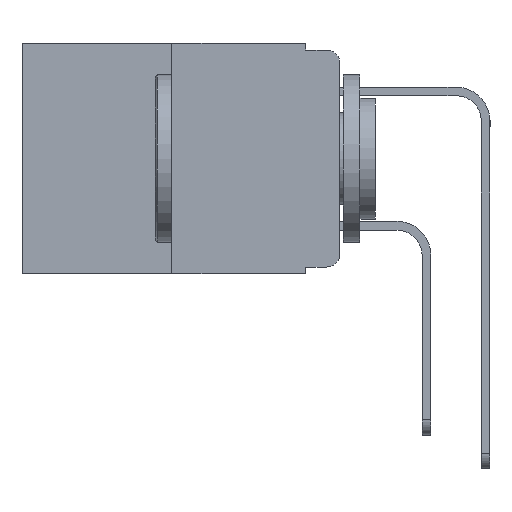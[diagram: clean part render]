
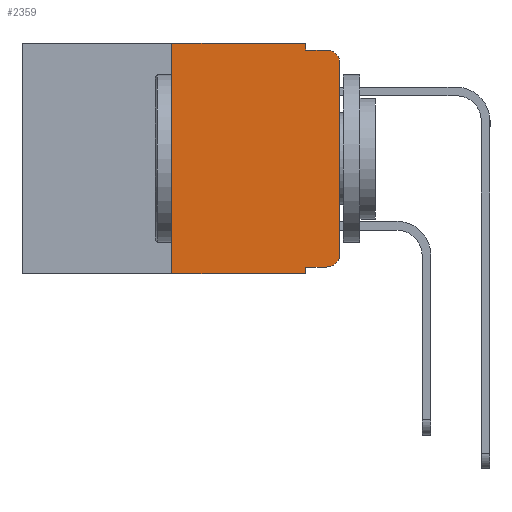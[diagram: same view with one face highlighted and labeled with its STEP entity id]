
A CAD part, left-side view. The second image highlights one B-rep face of the part: STEP entity #2359.
In plain terms, the highlighted planar face has unit normal (-1, 0, 0).
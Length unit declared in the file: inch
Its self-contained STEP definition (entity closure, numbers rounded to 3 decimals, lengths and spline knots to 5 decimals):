
#5 = CARTESIAN_POINT ( 'NONE',  ( 0., 0.051, -0.333 ) ) ;
#31 = VERTEX_POINT ( 'NONE', #13778 ) ;
#404 = LINE ( 'NONE', #16839, #7395 ) ;
#1077 = CARTESIAN_POINT ( 'NONE',  ( 0., 0.02, -0.333 ) ) ;
#1206 = ORIENTED_EDGE ( 'NONE', *, *, #13495, .T. ) ;
#1673 = VERTEX_POINT ( 'NONE', #5 ) ;
#1709 = VERTEX_POINT ( 'NONE', #17015 ) ;
#1797 = CARTESIAN_POINT ( 'NONE',  ( 0., 0.25, -0.343 ) ) ;
#1930 = VERTEX_POINT ( 'NONE', #12242 ) ;
#2124 = EDGE_CURVE ( 'NONE', #31, #9422, #9841, .T. ) ;
#2218 = CIRCLE ( 'NONE', #16726, 0.02 ) ;
#2359 = ADVANCED_FACE ( 'NONE', ( #3169 ), #11606, .F. ) ;
#2399 = CARTESIAN_POINT ( 'NONE',  ( 0., 0.473, 0. ) ) ;
#2436 = DIRECTION ( 'NONE',  ( 1., 0., 0. ) ) ;
#2530 = VECTOR ( 'NONE', #5152, 39.37008 ) ;
#2601 = EDGE_CURVE ( 'NONE', #1673, #15178, #6934, .T. ) ;
#2686 = ORIENTED_EDGE ( 'NONE', *, *, #4987, .T. ) ;
#2982 = CARTESIAN_POINT ( 'NONE',  ( 0., 0.25, 0. ) ) ;
#3169 = FACE_OUTER_BOUND ( 'NONE', #14978, .T. ) ;
#3383 = DIRECTION ( 'NONE',  ( 0., 0., 1. ) ) ;
#3404 = DIRECTION ( 'NONE',  ( 0., 0., -1. ) ) ;
#3457 = LINE ( 'NONE', #8446, #13752 ) ;
#4270 = ORIENTED_EDGE ( 'NONE', *, *, #2601, .T. ) ;
#4441 = VERTEX_POINT ( 'NONE', #1797 ) ;
#4460 = CIRCLE ( 'NONE', #12005, 0.02 ) ;
#4987 = EDGE_CURVE ( 'NONE', #1709, #9422, #2218, .T. ) ;
#5007 = VERTEX_POINT ( 'NONE', #14518 ) ;
#5067 = DIRECTION ( 'NONE',  ( 0., 0., -1. ) ) ;
#5077 = CARTESIAN_POINT ( 'NONE',  ( 0., 0.051, -0.01 ) ) ;
#5152 = DIRECTION ( 'NONE',  ( 0., -1., 0. ) ) ;
#5362 = VECTOR ( 'NONE', #13006, 39.37008 ) ;
#5490 = VECTOR ( 'NONE', #3383, 39.37008 ) ;
#5798 = ORIENTED_EDGE ( 'NONE', *, *, #11610, .F. ) ;
#6322 = DIRECTION ( 'NONE',  ( 0., -1., 0. ) ) ;
#6460 = DIRECTION ( 'NONE',  ( -1., 0., 0. ) ) ;
#6934 = LINE ( 'NONE', #14361, #10056 ) ;
#6973 = CARTESIAN_POINT ( 'NONE',  ( 0., 0.051, -0.343 ) ) ;
#7395 = VECTOR ( 'NONE', #5067, 39.37008 ) ;
#7733 = EDGE_CURVE ( 'NONE', #14013, #1709, #12569, .T. ) ;
#7748 = CARTESIAN_POINT ( 'NONE',  ( 0., 0.473, 0. ) ) ;
#7845 = EDGE_CURVE ( 'NONE', #1673, #14647, #404, .T. ) ;
#7867 = LINE ( 'NONE', #2982, #14829 ) ;
#8128 = ORIENTED_EDGE ( 'NONE', *, *, #15922, .F. ) ;
#8321 = LINE ( 'NONE', #13346, #11854 ) ;
#8446 = CARTESIAN_POINT ( 'NONE',  ( 0., 0.051, 0. ) ) ;
#8754 = ORIENTED_EDGE ( 'NONE', *, *, #7733, .T. ) ;
#9156 = CARTESIAN_POINT ( 'NONE',  ( 0., 0., -0.313 ) ) ;
#9413 = AXIS2_PLACEMENT_3D ( 'NONE', #2399, #2436, #3404 ) ;
#9422 = VERTEX_POINT ( 'NONE', #16927 ) ;
#9841 = LINE ( 'NONE', #5077, #2530 ) ;
#9882 = DIRECTION ( 'NONE',  ( 0., 0., 1. ) ) ;
#10056 = VECTOR ( 'NONE', #6322, 39.37008 ) ;
#11233 = LINE ( 'NONE', #7748, #5362 ) ;
#11266 = ORIENTED_EDGE ( 'NONE', *, *, #11620, .T. ) ;
#11606 = PLANE ( 'NONE',  #9413 ) ;
#11610 = EDGE_CURVE ( 'NONE', #5007, #1930, #11233, .T. ) ;
#11620 = EDGE_CURVE ( 'NONE', #15178, #14013, #4460, .T. ) ;
#11854 = VECTOR ( 'NONE', #14631, 39.37008 ) ;
#12005 = AXIS2_PLACEMENT_3D ( 'NONE', #14334, #6460, #15615 ) ;
#12242 = CARTESIAN_POINT ( 'NONE',  ( 0., 0.051, 0. ) ) ;
#12499 = EDGE_CURVE ( 'NONE', #4441, #5007, #7867, .T. ) ;
#12569 = LINE ( 'NONE', #12840, #5490 ) ;
#12840 = CARTESIAN_POINT ( 'NONE',  ( 0., 0., 0. ) ) ;
#13006 = DIRECTION ( 'NONE',  ( 0., -1., 0. ) ) ;
#13346 = CARTESIAN_POINT ( 'NONE',  ( 0., 0.473, -0.343 ) ) ;
#13495 = EDGE_CURVE ( 'NONE', #4441, #14647, #8321, .T. ) ;
#13644 = DIRECTION ( 'NONE',  ( 0., 0., -1. ) ) ;
#13752 = VECTOR ( 'NONE', #13644, 39.37008 ) ;
#13778 = CARTESIAN_POINT ( 'NONE',  ( 0., 0.051, -0.01 ) ) ;
#14013 = VERTEX_POINT ( 'NONE', #9156 ) ;
#14334 = CARTESIAN_POINT ( 'NONE',  ( 0., 0.02, -0.313 ) ) ;
#14361 = CARTESIAN_POINT ( 'NONE',  ( 0., 0.051, -0.333 ) ) ;
#14518 = CARTESIAN_POINT ( 'NONE',  ( 0., 0.25, 0. ) ) ;
#14631 = DIRECTION ( 'NONE',  ( 0., -1., 0. ) ) ;
#14647 = VERTEX_POINT ( 'NONE', #6973 ) ;
#14672 = ORIENTED_EDGE ( 'NONE', *, *, #2124, .F. ) ;
#14829 = VECTOR ( 'NONE', #9882, 39.37008 ) ;
#14978 = EDGE_LOOP ( 'NONE', ( #8754, #2686, #14672, #8128, #5798, #16461, #1206, #16271, #4270, #11266 ) ) ;
#15178 = VERTEX_POINT ( 'NONE', #1077 ) ;
#15615 = DIRECTION ( 'NONE',  ( 0., 0., -1. ) ) ;
#15922 = EDGE_CURVE ( 'NONE', #1930, #31, #3457, .T. ) ;
#16121 = DIRECTION ( 'NONE',  ( -1., 0., 0. ) ) ;
#16243 = CARTESIAN_POINT ( 'NONE',  ( 0., 0.02, -0.03 ) ) ;
#16271 = ORIENTED_EDGE ( 'NONE', *, *, #7845, .F. ) ;
#16424 = DIRECTION ( 'NONE',  ( 0., 0., -1. ) ) ;
#16461 = ORIENTED_EDGE ( 'NONE', *, *, #12499, .F. ) ;
#16726 = AXIS2_PLACEMENT_3D ( 'NONE', #16243, #16121, #16424 ) ;
#16839 = CARTESIAN_POINT ( 'NONE',  ( 0., 0.051, 0. ) ) ;
#16927 = CARTESIAN_POINT ( 'NONE',  ( 0., 0.02, -0.01 ) ) ;
#17015 = CARTESIAN_POINT ( 'NONE',  ( 0., 0., -0.03 ) ) ;
